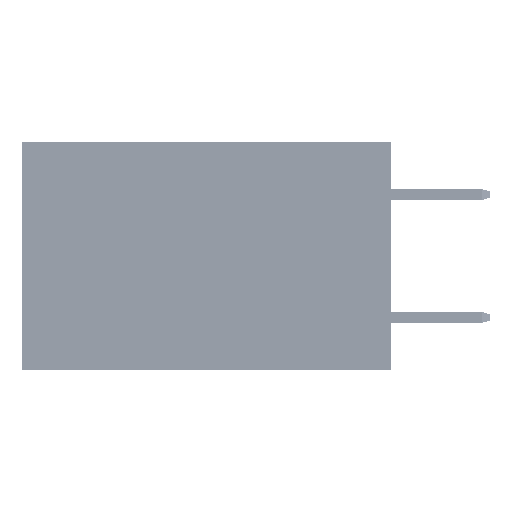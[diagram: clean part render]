
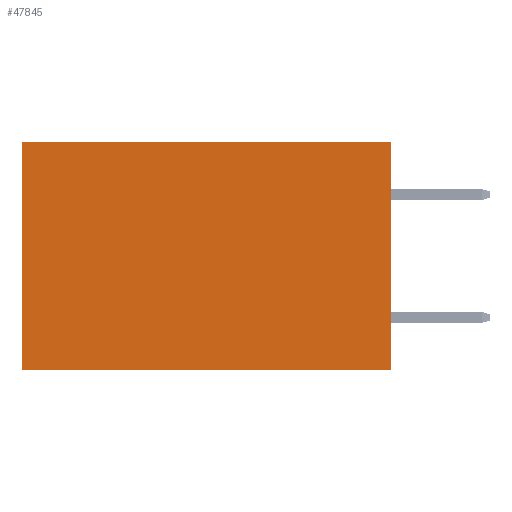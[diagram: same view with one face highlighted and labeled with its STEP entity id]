
A CAD part, left-side view. The second image highlights one B-rep face of the part: STEP entity #47845.
In plain terms, the highlighted planar face has unit normal (-1, 0, 0).
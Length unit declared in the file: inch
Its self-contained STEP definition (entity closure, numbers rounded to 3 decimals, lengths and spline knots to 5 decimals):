
#652 = VECTOR ( 'NONE', #4090, 39.37008 ) ;
#1473 = FACE_OUTER_BOUND ( 'NONE', #2075, .T. ) ;
#1588 = CARTESIAN_POINT ( 'NONE',  ( 0.2875, 0., -0.37 ) ) ;
#1605 = VERTEX_POINT ( 'NONE', #1588 ) ;
#2036 = ORIENTED_EDGE ( 'NONE', *, *, #15272, .F. ) ;
#2075 = EDGE_LOOP ( 'NONE', ( #21581, #2036, #15255, #12037 ) ) ;
#4090 = DIRECTION ( 'NONE',  ( 0., 1., 0. ) ) ;
#5931 = DIRECTION ( 'NONE',  ( 0., 0., -1. ) ) ;
#9584 = VERTEX_POINT ( 'NONE', #30226 ) ;
#9650 = CARTESIAN_POINT ( 'NONE',  ( 0.2875, 0., 0. ) ) ;
#12037 = ORIENTED_EDGE ( 'NONE', *, *, #49360, .T. ) ;
#13446 = LINE ( 'NONE', #38797, #652 ) ;
#13864 = LINE ( 'NONE', #24270, #39437 ) ;
#14676 = VECTOR ( 'NONE', #39234, 39.37008 ) ;
#15255 = ORIENTED_EDGE ( 'NONE', *, *, #18085, .F. ) ;
#15272 = EDGE_CURVE ( 'NONE', #1605, #44455, #47475, .T. ) ;
#17350 = CARTESIAN_POINT ( 'NONE',  ( 0.2875, 0.6, -0.37 ) ) ;
#17796 = DIRECTION ( 'NONE',  ( 1., 0., 0. ) ) ;
#18085 = EDGE_CURVE ( 'NONE', #42209, #1605, #13864, .T. ) ;
#21581 = ORIENTED_EDGE ( 'NONE', *, *, #43288, .T. ) ;
#21992 = CARTESIAN_POINT ( 'NONE',  ( 0.2875, 0., 0. ) ) ;
#24270 = CARTESIAN_POINT ( 'NONE',  ( 0.2875, 0., 0. ) ) ;
#28489 = DIRECTION ( 'NONE',  ( 0., 0., -1. ) ) ;
#29240 = CARTESIAN_POINT ( 'NONE',  ( 0.2875, 0.6, 0. ) ) ;
#30226 = CARTESIAN_POINT ( 'NONE',  ( 0.2875, 0.6, 0. ) ) ;
#30529 = VECTOR ( 'NONE', #5931, 39.37008 ) ;
#35311 = CARTESIAN_POINT ( 'NONE',  ( 0.2875, 0., -0.37 ) ) ;
#36681 = AXIS2_PLACEMENT_3D ( 'NONE', #9650, #17796, #49913 ) ;
#38797 = CARTESIAN_POINT ( 'NONE',  ( 0.2875, 0., 0. ) ) ;
#39234 = DIRECTION ( 'NONE',  ( 0., 1., 0. ) ) ;
#39437 = VECTOR ( 'NONE', #28489, 39.37008 ) ;
#40898 = LINE ( 'NONE', #29240, #30529 ) ;
#41145 = PLANE ( 'NONE',  #36681 ) ;
#42209 = VERTEX_POINT ( 'NONE', #21992 ) ;
#43288 = EDGE_CURVE ( 'NONE', #9584, #44455, #40898, .T. ) ;
#44455 = VERTEX_POINT ( 'NONE', #17350 ) ;
#47475 = LINE ( 'NONE', #35311, #14676 ) ;
#47845 = ADVANCED_FACE ( 'NONE', ( #1473 ), #41145, .F. ) ;
#49360 = EDGE_CURVE ( 'NONE', #42209, #9584, #13446, .T. ) ;
#49913 = DIRECTION ( 'NONE',  ( 0., 0., -1. ) ) ;
